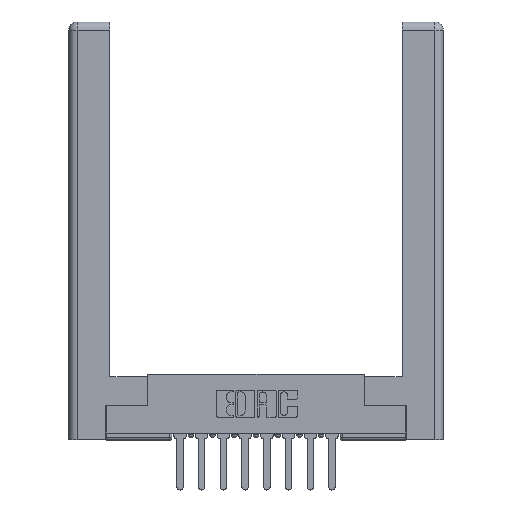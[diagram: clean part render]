
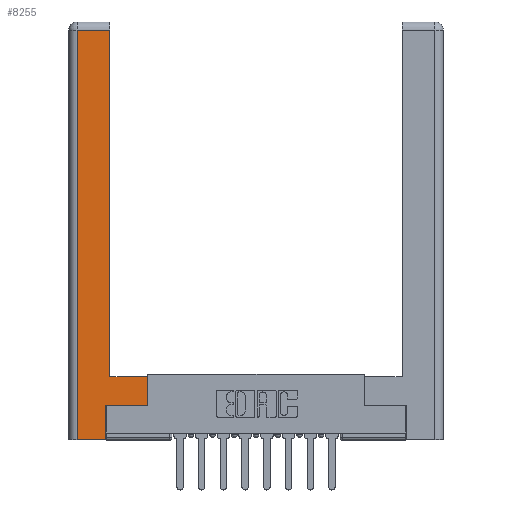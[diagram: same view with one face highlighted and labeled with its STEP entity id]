
A CAD part, top view. The second image highlights one B-rep face of the part: STEP entity #8255.
In plain terms, the highlighted planar face has unit normal (0, 0, 1).
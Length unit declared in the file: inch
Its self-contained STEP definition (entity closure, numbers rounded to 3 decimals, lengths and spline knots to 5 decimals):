
#148 = CARTESIAN_POINT ( 'NONE',  ( 0.265, 0.245, 0. ) ) ;
#205 = CARTESIAN_POINT ( 'NONE',  ( 0.0615, 2.94, 0. ) ) ;
#413 = CARTESIAN_POINT ( 'NONE',  ( 0., 0., 0. ) ) ;
#441 = VERTEX_POINT ( 'NONE', #9722 ) ;
#702 = CARTESIAN_POINT ( 'NONE',  ( 0.565, 0.45, 0. ) ) ;
#769 = ORIENTED_EDGE ( 'NONE', *, *, #1431, .T. ) ;
#927 = DIRECTION ( 'NONE',  ( 1., 0., 0. ) ) ;
#962 = ORIENTED_EDGE ( 'NONE', *, *, #6684, .T. ) ;
#1232 = VECTOR ( 'NONE', #6979, 39.37008 ) ;
#1431 = EDGE_CURVE ( 'NONE', #8115, #12538, #6220, .T. ) ;
#1499 = DIRECTION ( 'NONE',  ( 0., 1., 0. ) ) ;
#1541 = CARTESIAN_POINT ( 'NONE',  ( 0.0615, 0., 0. ) ) ;
#1877 = AXIS2_PLACEMENT_3D ( 'NONE', #413, #5692, #6682 ) ;
#1910 = ORIENTED_EDGE ( 'NONE', *, *, #7620, .T. ) ;
#2026 = CARTESIAN_POINT ( 'NONE',  ( 0.295, 2.94, 0. ) ) ;
#2398 = PLANE ( 'NONE',  #1877 ) ;
#2418 = EDGE_CURVE ( 'NONE', #13804, #10659, #9034, .T. ) ;
#2443 = ORIENTED_EDGE ( 'NONE', *, *, #4747, .T. ) ;
#2606 = ORIENTED_EDGE ( 'NONE', *, *, #2418, .T. ) ;
#2654 = ORIENTED_EDGE ( 'NONE', *, *, #11634, .T. ) ;
#2696 = CARTESIAN_POINT ( 'NONE',  ( 0.295, 0.45, 0. ) ) ;
#2771 = CARTESIAN_POINT ( 'NONE',  ( 0.265, 0., 0. ) ) ;
#2806 = VERTEX_POINT ( 'NONE', #10866 ) ;
#2881 = DIRECTION ( 'NONE',  ( 0., -1., 0. ) ) ;
#2931 = CARTESIAN_POINT ( 'NONE',  ( 0.565, 0.245, 0. ) ) ;
#2975 = VECTOR ( 'NONE', #10945, 39.37008 ) ;
#3691 = LINE ( 'NONE', #6775, #13375 ) ;
#4231 = DIRECTION ( 'NONE',  ( 0., 1., 0. ) ) ;
#4747 = EDGE_CURVE ( 'NONE', #10659, #441, #8994, .T. ) ;
#5692 = DIRECTION ( 'NONE',  ( 0., 0., -1. ) ) ;
#6220 = LINE ( 'NONE', #10521, #12104 ) ;
#6346 = VECTOR ( 'NONE', #4231, 39.37008 ) ;
#6589 = VERTEX_POINT ( 'NONE', #702 ) ;
#6682 = DIRECTION ( 'NONE',  ( -1., 0., 0. ) ) ;
#6684 = EDGE_CURVE ( 'NONE', #7550, #13804, #10716, .T. ) ;
#6775 = CARTESIAN_POINT ( 'NONE',  ( 0.265, 0.245, 0. ) ) ;
#6871 = ORIENTED_EDGE ( 'NONE', *, *, #11515, .T. ) ;
#6979 = DIRECTION ( 'NONE',  ( -1., 0., 0. ) ) ;
#7550 = VERTEX_POINT ( 'NONE', #11586 ) ;
#7558 = DIRECTION ( 'NONE',  ( 0., 1., 0. ) ) ;
#7614 = CARTESIAN_POINT ( 'NONE',  ( 0.565, 0.45, 0. ) ) ;
#7620 = EDGE_CURVE ( 'NONE', #12538, #6589, #11718, .T. ) ;
#8115 = VERTEX_POINT ( 'NONE', #148 ) ;
#8255 = ADVANCED_FACE ( 'NONE', ( #12048 ), #2398, .F. ) ;
#8412 = ORIENTED_EDGE ( 'NONE', *, *, #11552, .T. ) ;
#8564 = EDGE_LOOP ( 'NONE', ( #962, #2606, #2443, #2654, #6871, #769, #1910, #8412 ) ) ;
#8994 = LINE ( 'NONE', #1541, #10803 ) ;
#9034 = LINE ( 'NONE', #13338, #2975 ) ;
#9722 = CARTESIAN_POINT ( 'NONE',  ( 0.0615, 0., 0. ) ) ;
#10238 = VECTOR ( 'NONE', #10295, 39.37008 ) ;
#10295 = DIRECTION ( 'NONE',  ( 1., 0., 0. ) ) ;
#10515 = LINE ( 'NONE', #2771, #10238 ) ;
#10521 = CARTESIAN_POINT ( 'NONE',  ( 0.565, 0.245, 0. ) ) ;
#10659 = VERTEX_POINT ( 'NONE', #205 ) ;
#10716 = LINE ( 'NONE', #11772, #6346 ) ;
#10803 = VECTOR ( 'NONE', #2881, 39.37008 ) ;
#10866 = CARTESIAN_POINT ( 'NONE',  ( 0.265, 0., 0. ) ) ;
#10945 = DIRECTION ( 'NONE',  ( -1., 0., 0. ) ) ;
#11515 = EDGE_CURVE ( 'NONE', #2806, #8115, #3691, .T. ) ;
#11552 = EDGE_CURVE ( 'NONE', #6589, #7550, #12344, .T. ) ;
#11586 = CARTESIAN_POINT ( 'NONE',  ( 0.295, 0.45, 0. ) ) ;
#11634 = EDGE_CURVE ( 'NONE', #441, #2806, #10515, .T. ) ;
#11718 = LINE ( 'NONE', #7614, #12896 ) ;
#11772 = CARTESIAN_POINT ( 'NONE',  ( 0.295, 3., 0. ) ) ;
#12048 = FACE_OUTER_BOUND ( 'NONE', #8564, .T. ) ;
#12104 = VECTOR ( 'NONE', #927, 39.37008 ) ;
#12344 = LINE ( 'NONE', #2696, #1232 ) ;
#12538 = VERTEX_POINT ( 'NONE', #2931 ) ;
#12896 = VECTOR ( 'NONE', #7558, 39.37008 ) ;
#13338 = CARTESIAN_POINT ( 'NONE',  ( 0.0615, 2.94, 0. ) ) ;
#13375 = VECTOR ( 'NONE', #1499, 39.37008 ) ;
#13804 = VERTEX_POINT ( 'NONE', #2026 ) ;
